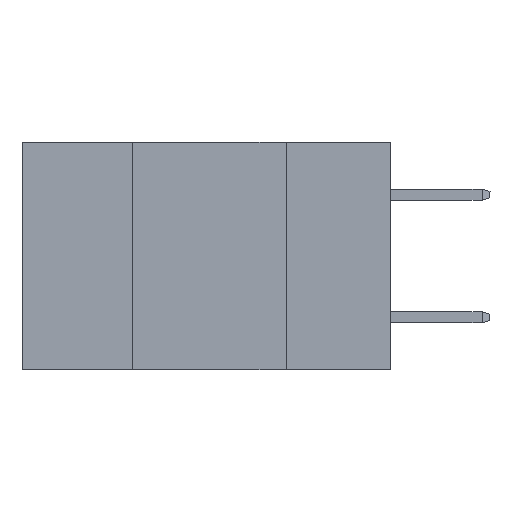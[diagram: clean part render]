
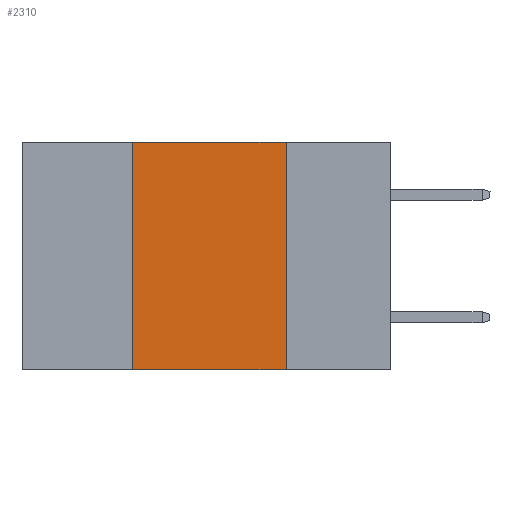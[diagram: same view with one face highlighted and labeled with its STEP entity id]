
A CAD part, left-side view. The second image highlights one B-rep face of the part: STEP entity #2310.
In plain terms, the highlighted planar face has unit normal (-1, 0, 0).
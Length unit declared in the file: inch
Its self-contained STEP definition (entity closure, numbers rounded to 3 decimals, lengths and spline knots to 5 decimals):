
#67 = LINE ( 'NONE', #7975, #10274 ) ;
#640 = VERTEX_POINT ( 'NONE', #12957 ) ;
#840 = AXIS2_PLACEMENT_3D ( 'NONE', #15225, #12738, #5098 ) ;
#1628 = DIRECTION ( 'NONE',  ( 0., 0., -1. ) ) ;
#1791 = EDGE_CURVE ( 'NONE', #640, #7637, #6768, .T. ) ;
#2310 = ADVANCED_FACE ( 'NONE', ( #14886 ), #11484, .F. ) ;
#2592 = EDGE_CURVE ( 'NONE', #8760, #6771, #7984, .T. ) ;
#2685 = ORIENTED_EDGE ( 'NONE', *, *, #2592, .F. ) ;
#2843 = DIRECTION ( 'NONE',  ( 0., 0., 1. ) ) ;
#5098 = DIRECTION ( 'NONE',  ( 0., 0., -1. ) ) ;
#5349 = DIRECTION ( 'NONE',  ( 0., -1., 0. ) ) ;
#5948 = VECTOR ( 'NONE', #2843, 39.37008 ) ;
#6768 = LINE ( 'NONE', #11876, #5948 ) ;
#6771 = VERTEX_POINT ( 'NONE', #8601 ) ;
#7030 = EDGE_LOOP ( 'NONE', ( #2685, #7416, #7816, #9039 ) ) ;
#7416 = ORIENTED_EDGE ( 'NONE', *, *, #14939, .F. ) ;
#7637 = VERTEX_POINT ( 'NONE', #15946 ) ;
#7816 = ORIENTED_EDGE ( 'NONE', *, *, #1791, .F. ) ;
#7975 = CARTESIAN_POINT ( 'NONE',  ( 0., 0.6, -0.37 ) ) ;
#7984 = LINE ( 'NONE', #9518, #14279 ) ;
#8601 = CARTESIAN_POINT ( 'NONE',  ( 0., 0.17, -0.37 ) ) ;
#8760 = VERTEX_POINT ( 'NONE', #15527 ) ;
#9039 = ORIENTED_EDGE ( 'NONE', *, *, #10882, .T. ) ;
#9518 = CARTESIAN_POINT ( 'NONE',  ( 0., 0.17, 0. ) ) ;
#10274 = VECTOR ( 'NONE', #5349, 39.37008 ) ;
#10882 = EDGE_CURVE ( 'NONE', #640, #6771, #67, .T. ) ;
#11153 = DIRECTION ( 'NONE',  ( 0., -1., 0. ) ) ;
#11484 = PLANE ( 'NONE',  #840 ) ;
#11876 = CARTESIAN_POINT ( 'NONE',  ( 0., 0.42, 0. ) ) ;
#12738 = DIRECTION ( 'NONE',  ( 1., 0., 0. ) ) ;
#12842 = VECTOR ( 'NONE', #11153, 39.37008 ) ;
#12957 = CARTESIAN_POINT ( 'NONE',  ( 0., 0.42, -0.37 ) ) ;
#13627 = LINE ( 'NONE', #13662, #12842 ) ;
#13662 = CARTESIAN_POINT ( 'NONE',  ( 0., 0.6, 0. ) ) ;
#14279 = VECTOR ( 'NONE', #1628, 39.37008 ) ;
#14886 = FACE_OUTER_BOUND ( 'NONE', #7030, .T. ) ;
#14939 = EDGE_CURVE ( 'NONE', #7637, #8760, #13627, .T. ) ;
#15225 = CARTESIAN_POINT ( 'NONE',  ( 0., 0.6, 0. ) ) ;
#15527 = CARTESIAN_POINT ( 'NONE',  ( 0., 0.17, 0. ) ) ;
#15946 = CARTESIAN_POINT ( 'NONE',  ( 0., 0.42, 0. ) ) ;
